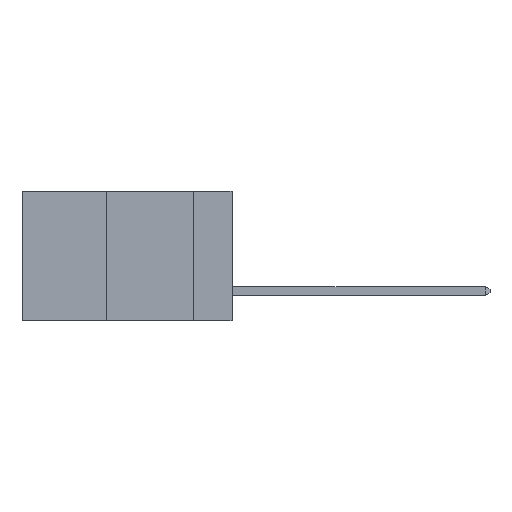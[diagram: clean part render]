
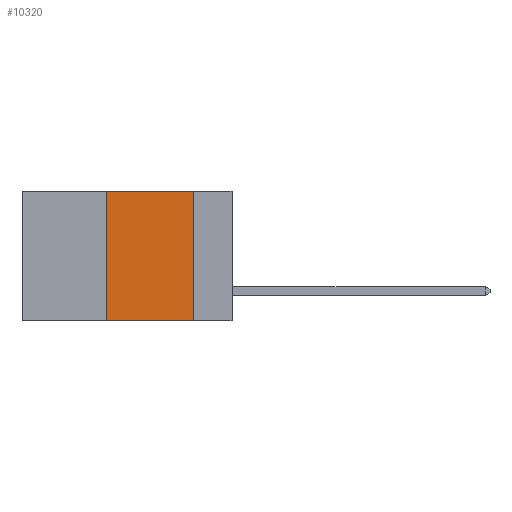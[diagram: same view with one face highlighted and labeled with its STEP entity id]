
A CAD part, left-side view. The second image highlights one B-rep face of the part: STEP entity #10320.
In plain terms, the highlighted planar face has unit normal (-1, 0, 0).
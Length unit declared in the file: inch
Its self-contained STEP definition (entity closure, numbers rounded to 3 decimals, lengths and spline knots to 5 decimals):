
#150 = EDGE_CURVE ( 'NONE', #24588, #11878, #18855, .T. ) ;
#665 = DIRECTION ( 'NONE',  ( 0., -1., 0. ) ) ;
#922 = CARTESIAN_POINT ( 'NONE',  ( 0., 0.36, -0.37 ) ) ;
#1335 = DIRECTION ( 'NONE',  ( 0., 0., 1. ) ) ;
#1449 = EDGE_CURVE ( 'NONE', #6384, #11878, #20250, .T. ) ;
#2068 = DIRECTION ( 'NONE',  ( 0., 0., -1. ) ) ;
#3124 = FACE_OUTER_BOUND ( 'NONE', #26069, .T. ) ;
#3157 = LINE ( 'NONE', #15341, #10375 ) ;
#3652 = VERTEX_POINT ( 'NONE', #7161 ) ;
#6015 = VECTOR ( 'NONE', #2068, 39.37008 ) ;
#6384 = VERTEX_POINT ( 'NONE', #922 ) ;
#7022 = CARTESIAN_POINT ( 'NONE',  ( 0., 0.6, 0. ) ) ;
#7161 = CARTESIAN_POINT ( 'NONE',  ( 0., 0.36, 0. ) ) ;
#8262 = ORIENTED_EDGE ( 'NONE', *, *, #16775, .F. ) ;
#8592 = VECTOR ( 'NONE', #1335, 39.37008 ) ;
#9904 = EDGE_CURVE ( 'NONE', #3652, #24588, #3157, .T. ) ;
#10320 = ADVANCED_FACE ( 'NONE', ( #3124 ), #11903, .F. ) ;
#10375 = VECTOR ( 'NONE', #665, 39.37008 ) ;
#11878 = VERTEX_POINT ( 'NONE', #15233 ) ;
#11903 = PLANE ( 'NONE',  #23585 ) ;
#13548 = CARTESIAN_POINT ( 'NONE',  ( 0., 0.36, 0. ) ) ;
#15233 = CARTESIAN_POINT ( 'NONE',  ( 0., 0.11, -0.37 ) ) ;
#15341 = CARTESIAN_POINT ( 'NONE',  ( 0., 0.6, 0. ) ) ;
#16141 = ORIENTED_EDGE ( 'NONE', *, *, #150, .F. ) ;
#16771 = DIRECTION ( 'NONE',  ( 0., 0., -1. ) ) ;
#16775 = EDGE_CURVE ( 'NONE', #6384, #3652, #26793, .T. ) ;
#18855 = LINE ( 'NONE', #28461, #6015 ) ;
#20250 = LINE ( 'NONE', #22844, #26443 ) ;
#22511 = ORIENTED_EDGE ( 'NONE', *, *, #1449, .T. ) ;
#22750 = DIRECTION ( 'NONE',  ( 0., -1., 0. ) ) ;
#22844 = CARTESIAN_POINT ( 'NONE',  ( 0., 0.6, -0.37 ) ) ;
#23585 = AXIS2_PLACEMENT_3D ( 'NONE', #7022, #30690, #16771 ) ;
#24068 = CARTESIAN_POINT ( 'NONE',  ( 0., 0.11, 0. ) ) ;
#24588 = VERTEX_POINT ( 'NONE', #24068 ) ;
#26069 = EDGE_LOOP ( 'NONE', ( #16141, #26862, #8262, #22511 ) ) ;
#26443 = VECTOR ( 'NONE', #22750, 39.37008 ) ;
#26793 = LINE ( 'NONE', #13548, #8592 ) ;
#26862 = ORIENTED_EDGE ( 'NONE', *, *, #9904, .F. ) ;
#28461 = CARTESIAN_POINT ( 'NONE',  ( 0., 0.11, 0. ) ) ;
#30690 = DIRECTION ( 'NONE',  ( 1., 0., 0. ) ) ;
